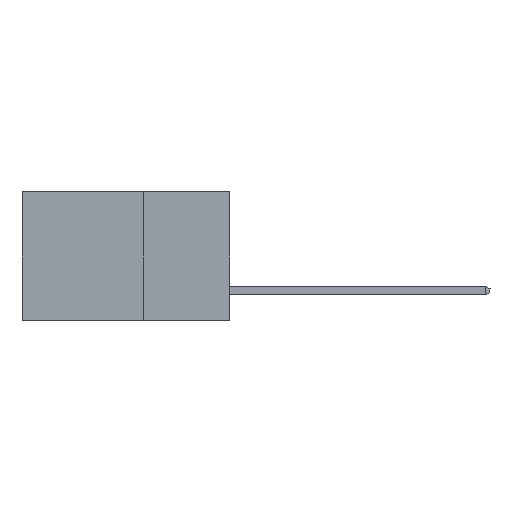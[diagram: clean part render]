
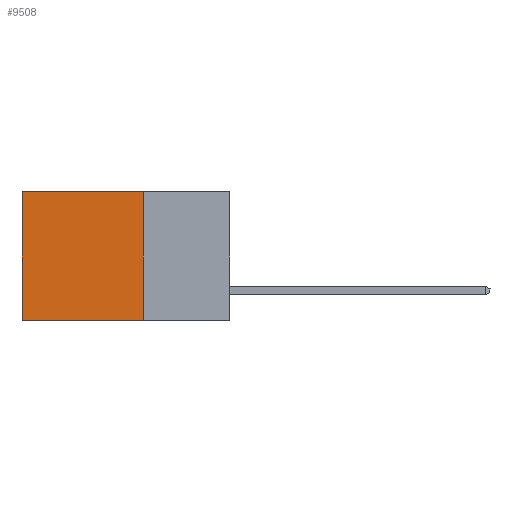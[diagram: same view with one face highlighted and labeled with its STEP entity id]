
A CAD part, left-side view. The second image highlights one B-rep face of the part: STEP entity #9508.
In plain terms, the highlighted planar face has unit normal (-1, 0, 0).
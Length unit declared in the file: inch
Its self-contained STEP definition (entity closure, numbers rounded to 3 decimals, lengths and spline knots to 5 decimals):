
#1001 = DIRECTION ( 'NONE',  ( 0., 0., -1. ) ) ;
#1688 = VECTOR ( 'NONE', #3221, 39.37008 ) ;
#2199 = EDGE_CURVE ( 'NONE', #8394, #16904, #4697, .T. ) ;
#2482 = DIRECTION ( 'NONE',  ( 1., 0., 0. ) ) ;
#2993 = DIRECTION ( 'NONE',  ( 0., 0., -1. ) ) ;
#3052 = CARTESIAN_POINT ( 'NONE',  ( 0.2615, 0.25, 0. ) ) ;
#3221 = DIRECTION ( 'NONE',  ( 0., 1., 0. ) ) ;
#4028 = ORIENTED_EDGE ( 'NONE', *, *, #4208, .T. ) ;
#4208 = EDGE_CURVE ( 'NONE', #4225, #8394, #5937, .T. ) ;
#4225 = VERTEX_POINT ( 'NONE', #16206 ) ;
#4338 = DIRECTION ( 'NONE',  ( 0., 1., 0. ) ) ;
#4615 = VECTOR ( 'NONE', #10186, 39.37008 ) ;
#4697 = LINE ( 'NONE', #11607, #14144 ) ;
#4801 = ORIENTED_EDGE ( 'NONE', *, *, #18626, .F. ) ;
#4926 = ORIENTED_EDGE ( 'NONE', *, *, #20975, .F. ) ;
#5754 = CARTESIAN_POINT ( 'NONE',  ( 0.2615, 0.25, -0.37 ) ) ;
#5937 = LINE ( 'NONE', #3052, #17442 ) ;
#8394 = VERTEX_POINT ( 'NONE', #9112 ) ;
#9112 = CARTESIAN_POINT ( 'NONE',  ( 0.2615, 0.6, 0. ) ) ;
#9508 = ADVANCED_FACE ( 'NONE', ( #14800 ), #11303, .F. ) ;
#10186 = DIRECTION ( 'NONE',  ( 0., 0., -1. ) ) ;
#11303 = PLANE ( 'NONE',  #17203 ) ;
#11607 = CARTESIAN_POINT ( 'NONE',  ( 0.2615, 0.6, -0.37 ) ) ;
#12426 = EDGE_LOOP ( 'NONE', ( #17044, #4801, #4926, #4028 ) ) ;
#12664 = CARTESIAN_POINT ( 'NONE',  ( 0.2615, 0.25, -0.37 ) ) ;
#13683 = LINE ( 'NONE', #17293, #4615 ) ;
#14144 = VECTOR ( 'NONE', #2993, 39.37008 ) ;
#14558 = CARTESIAN_POINT ( 'NONE',  ( 0.2615, 0.6, -0.37 ) ) ;
#14800 = FACE_OUTER_BOUND ( 'NONE', #12426, .T. ) ;
#15731 = VERTEX_POINT ( 'NONE', #5754 ) ;
#16206 = CARTESIAN_POINT ( 'NONE',  ( 0.2615, 0.25, 0. ) ) ;
#16904 = VERTEX_POINT ( 'NONE', #14558 ) ;
#17044 = ORIENTED_EDGE ( 'NONE', *, *, #2199, .T. ) ;
#17203 = AXIS2_PLACEMENT_3D ( 'NONE', #12664, #2482, #1001 ) ;
#17293 = CARTESIAN_POINT ( 'NONE',  ( 0.2615, 0.25, -0.37 ) ) ;
#17442 = VECTOR ( 'NONE', #4338, 39.37008 ) ;
#18626 = EDGE_CURVE ( 'NONE', #15731, #16904, #18707, .T. ) ;
#18707 = LINE ( 'NONE', #22321, #1688 ) ;
#20975 = EDGE_CURVE ( 'NONE', #4225, #15731, #13683, .T. ) ;
#22321 = CARTESIAN_POINT ( 'NONE',  ( 0.2615, 0.25, -0.37 ) ) ;
